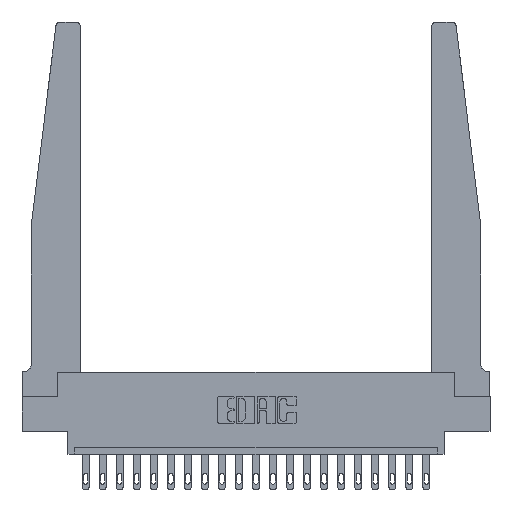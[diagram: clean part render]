
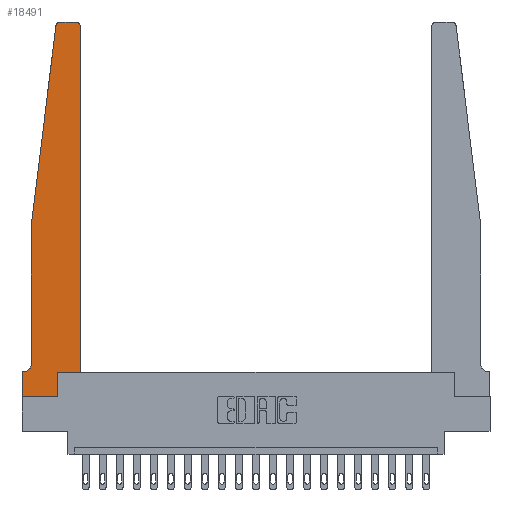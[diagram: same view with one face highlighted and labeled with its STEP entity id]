
A CAD part, top view. The second image highlights one B-rep face of the part: STEP entity #18491.
In plain terms, the highlighted planar face has unit normal (0, 0, 1).
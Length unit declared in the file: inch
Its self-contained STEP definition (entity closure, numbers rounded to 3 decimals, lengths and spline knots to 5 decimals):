
#54 = CARTESIAN_POINT ( 'NONE',  ( 0.425, 0.18, 0.37 ) ) ;
#555 = VECTOR ( 'NONE', #5524, 39.37008 ) ;
#771 = EDGE_CURVE ( 'NONE', #16922, #18946, #8742, .T. ) ;
#863 = VERTEX_POINT ( 'NONE', #11609 ) ;
#1626 = DIRECTION ( 'NONE',  ( 0., 0., 1. ) ) ;
#2033 = VERTEX_POINT ( 'NONE', #11400 ) ;
#2231 = EDGE_CURVE ( 'NONE', #20507, #6190, #20393, .T. ) ;
#2478 = LINE ( 'NONE', #8994, #15166 ) ;
#2537 = DIRECTION ( 'NONE',  ( 0., 0., 1. ) ) ;
#2594 = CARTESIAN_POINT ( 'NONE',  ( 0.24675, 2.72367, 0.37 ) ) ;
#2717 = DIRECTION ( 'NONE',  ( 0., -1., 0. ) ) ;
#2792 = CARTESIAN_POINT ( 'NONE',  ( 0.27653, 2.75, 0.37 ) ) ;
#3221 = CARTESIAN_POINT ( 'NONE',  ( 0.015, 0.2375, 0.37 ) ) ;
#3537 = CARTESIAN_POINT ( 'NONE',  ( 0.2605, 0.18, 0.37 ) ) ;
#4067 = FACE_OUTER_BOUND ( 'NONE', #15461, .T. ) ;
#4269 = EDGE_CURVE ( 'NONE', #2033, #13874, #2478, .T. ) ;
#5099 = LINE ( 'NONE', #17824, #15600 ) ;
#5275 = CARTESIAN_POINT ( 'NONE',  ( 0., 0., 0.37 ) ) ;
#5378 = ORIENTED_EDGE ( 'NONE', *, *, #18920, .T. ) ;
#5524 = DIRECTION ( 'NONE',  ( 0., -1., 0. ) ) ;
#5864 = ORIENTED_EDGE ( 'NONE', *, *, #12700, .T. ) ;
#5865 = DIRECTION ( 'NONE',  ( 0., 0., 1. ) ) ;
#5913 = LINE ( 'NONE', #20892, #19764 ) ;
#5935 = CARTESIAN_POINT ( 'NONE',  ( 0.395, 2.72, 0.37 ) ) ;
#5996 = VERTEX_POINT ( 'NONE', #16209 ) ;
#6190 = VERTEX_POINT ( 'NONE', #6700 ) ;
#6198 = CARTESIAN_POINT ( 'NONE',  ( 0.015, 0.1875, 0.37 ) ) ;
#6317 = ORIENTED_EDGE ( 'NONE', *, *, #7448, .T. ) ;
#6634 = DIRECTION ( 'NONE',  ( 1., 0., 0. ) ) ;
#6646 = EDGE_CURVE ( 'NONE', #18946, #863, #16822, .T. ) ;
#6700 = CARTESIAN_POINT ( 'NONE',  ( 0.425, 0.18, 0.37 ) ) ;
#6714 = AXIS2_PLACEMENT_3D ( 'NONE', #5935, #2537, #16963 ) ;
#6764 = ORIENTED_EDGE ( 'NONE', *, *, #20354, .T. ) ;
#6807 = AXIS2_PLACEMENT_3D ( 'NONE', #8348, #1626, #6634 ) ;
#7448 = EDGE_CURVE ( 'NONE', #12247, #5996, #5099, .T. ) ;
#7623 = DIRECTION ( 'NONE',  ( -1., 0., 0. ) ) ;
#7673 = CARTESIAN_POINT ( 'NONE',  ( 0., 0.1875, 0.37 ) ) ;
#7781 = AXIS2_PLACEMENT_3D ( 'NONE', #3221, #19158, #9642 ) ;
#8089 = ORIENTED_EDGE ( 'NONE', *, *, #771, .T. ) ;
#8189 = DIRECTION ( 'NONE',  ( 0., 1., 0. ) ) ;
#8299 = ORIENTED_EDGE ( 'NONE', *, *, #21011, .T. ) ;
#8348 = CARTESIAN_POINT ( 'NONE',  ( 0.27653, 2.72, 0.37 ) ) ;
#8355 = ORIENTED_EDGE ( 'NONE', *, *, #9917, .T. ) ;
#8622 = LINE ( 'NONE', #18015, #12972 ) ;
#8742 = LINE ( 'NONE', #20067, #555 ) ;
#8994 = CARTESIAN_POINT ( 'NONE',  ( 0.25, 2.75, 0.37 ) ) ;
#9642 = DIRECTION ( 'NONE',  ( -1., 0., 0. ) ) ;
#9917 = EDGE_CURVE ( 'NONE', #5996, #19215, #20457, .T. ) ;
#10049 = VECTOR ( 'NONE', #14150, 39.37008 ) ;
#10214 = DIRECTION ( 'NONE',  ( 1., 0., 0. ) ) ;
#10437 = VERTEX_POINT ( 'NONE', #6198 ) ;
#11400 = CARTESIAN_POINT ( 'NONE',  ( 0.395, 2.75, 0.37 ) ) ;
#11453 = ORIENTED_EDGE ( 'NONE', *, *, #2231, .T. ) ;
#11579 = VECTOR ( 'NONE', #2717, 39.37008 ) ;
#11609 = CARTESIAN_POINT ( 'NONE',  ( 0.2605, 0., 0.37 ) ) ;
#11713 = ORIENTED_EDGE ( 'NONE', *, *, #4269, .T. ) ;
#11736 = EDGE_CURVE ( 'NONE', #13874, #12247, #19792, .T. ) ;
#12137 = ORIENTED_EDGE ( 'NONE', *, *, #19589, .T. ) ;
#12247 = VERTEX_POINT ( 'NONE', #2594 ) ;
#12700 = EDGE_CURVE ( 'NONE', #863, #20507, #8622, .T. ) ;
#12972 = VECTOR ( 'NONE', #8189, 39.37008 ) ;
#13003 = DIRECTION ( 'NONE',  ( -0.122, -0.992, 0. ) ) ;
#13057 = LINE ( 'NONE', #54, #19041 ) ;
#13874 = VERTEX_POINT ( 'NONE', #2792 ) ;
#14150 = DIRECTION ( 'NONE',  ( 1., 0., 0. ) ) ;
#14932 = ORIENTED_EDGE ( 'NONE', *, *, #11736, .T. ) ;
#15166 = VECTOR ( 'NONE', #15485, 39.37008 ) ;
#15289 = CIRCLE ( 'NONE', #7781, 0.05 ) ;
#15308 = CARTESIAN_POINT ( 'NONE',  ( 0.065, 1.25, 0.37 ) ) ;
#15345 = CARTESIAN_POINT ( 'NONE',  ( 0., 0., 0.37 ) ) ;
#15461 = EDGE_LOOP ( 'NONE', ( #11713, #14932, #6317, #8355, #6764, #8299, #8089, #17769, #5864, #11453, #12137, #5378 ) ) ;
#15485 = DIRECTION ( 'NONE',  ( -1., 0., 0. ) ) ;
#15600 = VECTOR ( 'NONE', #13003, 39.37008 ) ;
#15920 = CIRCLE ( 'NONE', #6714, 0.03 ) ;
#16209 = CARTESIAN_POINT ( 'NONE',  ( 0.065, 1.25, 0.37 ) ) ;
#16797 = CARTESIAN_POINT ( 'NONE',  ( 0., 0.1875, 0.37 ) ) ;
#16822 = LINE ( 'NONE', #5275, #20724 ) ;
#16922 = VERTEX_POINT ( 'NONE', #16797 ) ;
#16963 = DIRECTION ( 'NONE',  ( 1., 0., 0. ) ) ;
#17769 = ORIENTED_EDGE ( 'NONE', *, *, #6646, .T. ) ;
#17824 = CARTESIAN_POINT ( 'NONE',  ( 0.065, 1.25, 0.37 ) ) ;
#17924 = VERTEX_POINT ( 'NONE', #18326 ) ;
#18015 = CARTESIAN_POINT ( 'NONE',  ( 0.2605, 0.18, 0.37 ) ) ;
#18326 = CARTESIAN_POINT ( 'NONE',  ( 0.425, 2.72, 0.37 ) ) ;
#18445 = CARTESIAN_POINT ( 'NONE',  ( 0.065, 0.2375, 0.37 ) ) ;
#18491 = ADVANCED_FACE ( 'NONE', ( #4067 ), #18821, .T. ) ;
#18821 = PLANE ( 'NONE',  #21049 ) ;
#18895 = CARTESIAN_POINT ( 'NONE',  ( 0.425, 0.18, 0.37 ) ) ;
#18920 = EDGE_CURVE ( 'NONE', #17924, #2033, #15920, .T. ) ;
#18946 = VERTEX_POINT ( 'NONE', #15345 ) ;
#19041 = VECTOR ( 'NONE', #19906, 39.37008 ) ;
#19158 = DIRECTION ( 'NONE',  ( 0., 0., -1. ) ) ;
#19215 = VERTEX_POINT ( 'NONE', #18445 ) ;
#19589 = EDGE_CURVE ( 'NONE', #6190, #17924, #13057, .T. ) ;
#19764 = VECTOR ( 'NONE', #7623, 39.37008 ) ;
#19792 = CIRCLE ( 'NONE', #6807, 0.03 ) ;
#19906 = DIRECTION ( 'NONE',  ( 0., 1., 0. ) ) ;
#20067 = CARTESIAN_POINT ( 'NONE',  ( 0., 0., 0.37 ) ) ;
#20354 = EDGE_CURVE ( 'NONE', #19215, #10437, #15289, .T. ) ;
#20393 = LINE ( 'NONE', #18895, #10049 ) ;
#20457 = LINE ( 'NONE', #15308, #11579 ) ;
#20507 = VERTEX_POINT ( 'NONE', #3537 ) ;
#20723 = DIRECTION ( 'NONE',  ( 1., 0., 0. ) ) ;
#20724 = VECTOR ( 'NONE', #10214, 39.37008 ) ;
#20892 = CARTESIAN_POINT ( 'NONE',  ( 0.065, 0.1875, 0.37 ) ) ;
#21011 = EDGE_CURVE ( 'NONE', #10437, #16922, #5913, .T. ) ;
#21049 = AXIS2_PLACEMENT_3D ( 'NONE', #7673, #5865, #20723 ) ;
